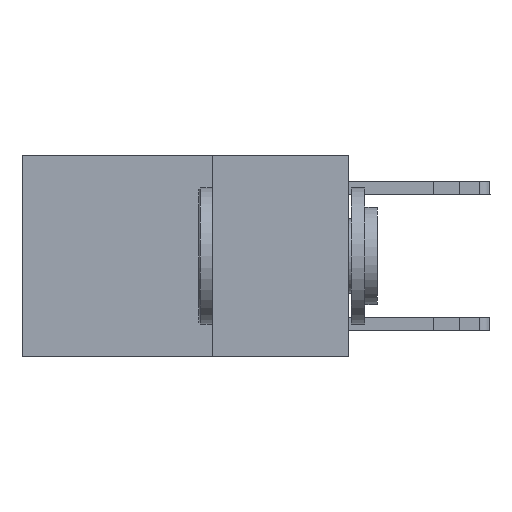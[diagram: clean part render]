
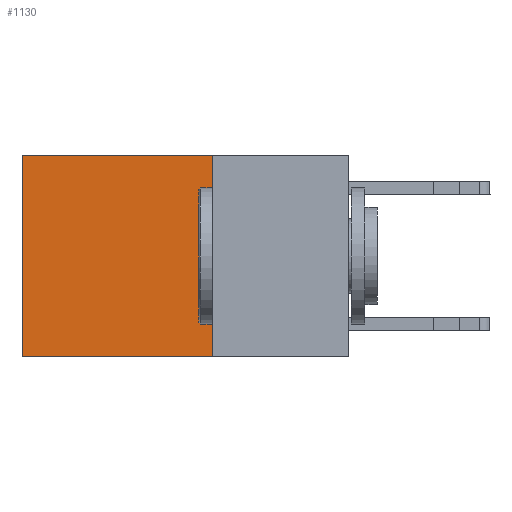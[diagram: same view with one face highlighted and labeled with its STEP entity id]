
A CAD part, left-side view. The second image highlights one B-rep face of the part: STEP entity #1130.
In plain terms, the highlighted planar face has unit normal (-1, 0, 0).
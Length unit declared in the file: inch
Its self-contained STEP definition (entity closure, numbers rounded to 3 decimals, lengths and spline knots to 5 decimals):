
#1130 = ADVANCED_FACE ( 'NONE', ( #16677 ), #18340, .F. ) ;
#1620 = VECTOR ( 'NONE', #2040, 39.37008 ) ;
#2040 = DIRECTION ( 'NONE',  ( 0., 1., 0. ) ) ;
#2445 = EDGE_CURVE ( 'NONE', #8718, #11183, #16682, .T. ) ;
#3687 = CARTESIAN_POINT ( 'NONE',  ( 0.2625, 0.25, 0. ) ) ;
#5493 = VECTOR ( 'NONE', #14936, 39.37008 ) ;
#5847 = LINE ( 'NONE', #10665, #11157 ) ;
#6739 = DIRECTION ( 'NONE',  ( 0., 0., -1. ) ) ;
#6787 = CARTESIAN_POINT ( 'NONE',  ( 0.2625, 0.25, -0.37 ) ) ;
#7245 = EDGE_CURVE ( 'NONE', #8718, #10848, #15139, .T. ) ;
#8511 = CARTESIAN_POINT ( 'NONE',  ( 0.2625, 0.25, 0. ) ) ;
#8718 = VERTEX_POINT ( 'NONE', #13950 ) ;
#9187 = EDGE_CURVE ( 'NONE', #11183, #9757, #5847, .T. ) ;
#9757 = VERTEX_POINT ( 'NONE', #12724 ) ;
#10073 = DIRECTION ( 'NONE',  ( 1., 0., 0. ) ) ;
#10665 = CARTESIAN_POINT ( 'NONE',  ( 0.2625, 0.6, 0. ) ) ;
#10848 = VERTEX_POINT ( 'NONE', #6787 ) ;
#11157 = VECTOR ( 'NONE', #17040, 39.37008 ) ;
#11183 = VERTEX_POINT ( 'NONE', #17638 ) ;
#11897 = CARTESIAN_POINT ( 'NONE',  ( 0.2625, 0.25, 0. ) ) ;
#12724 = CARTESIAN_POINT ( 'NONE',  ( 0.2625, 0.6, -0.37 ) ) ;
#13046 = VECTOR ( 'NONE', #18054, 39.37008 ) ;
#13950 = CARTESIAN_POINT ( 'NONE',  ( 0.2625, 0.25, 0. ) ) ;
#14936 = DIRECTION ( 'NONE',  ( 0., 0., -1. ) ) ;
#15139 = LINE ( 'NONE', #8511, #5493 ) ;
#16282 = LINE ( 'NONE', #17949, #13046 ) ;
#16401 = EDGE_CURVE ( 'NONE', #10848, #9757, #16282, .T. ) ;
#16658 = ORIENTED_EDGE ( 'NONE', *, *, #16401, .F. ) ;
#16677 = FACE_OUTER_BOUND ( 'NONE', #17696, .T. ) ;
#16682 = LINE ( 'NONE', #11897, #1620 ) ;
#17040 = DIRECTION ( 'NONE',  ( 0., 0., -1. ) ) ;
#17638 = CARTESIAN_POINT ( 'NONE',  ( 0.2625, 0.6, 0. ) ) ;
#17696 = EDGE_LOOP ( 'NONE', ( #19803, #16658, #18875, #20115 ) ) ;
#17949 = CARTESIAN_POINT ( 'NONE',  ( 0.2625, 0.25, -0.37 ) ) ;
#18054 = DIRECTION ( 'NONE',  ( 0., 1., 0. ) ) ;
#18340 = PLANE ( 'NONE',  #20583 ) ;
#18875 = ORIENTED_EDGE ( 'NONE', *, *, #7245, .F. ) ;
#19803 = ORIENTED_EDGE ( 'NONE', *, *, #9187, .T. ) ;
#20115 = ORIENTED_EDGE ( 'NONE', *, *, #2445, .T. ) ;
#20583 = AXIS2_PLACEMENT_3D ( 'NONE', #3687, #10073, #6739 ) ;
